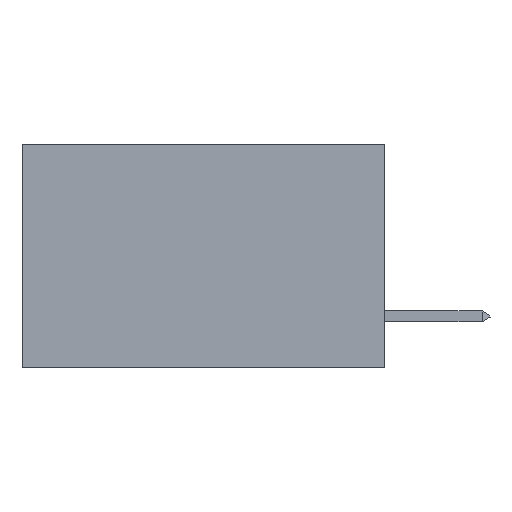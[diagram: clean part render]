
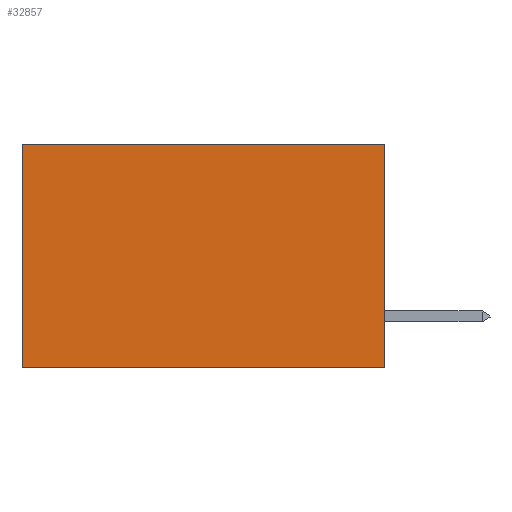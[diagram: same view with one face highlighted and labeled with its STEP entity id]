
A CAD part, left-side view. The second image highlights one B-rep face of the part: STEP entity #32857.
In plain terms, the highlighted planar face has unit normal (-1, 0, 0).
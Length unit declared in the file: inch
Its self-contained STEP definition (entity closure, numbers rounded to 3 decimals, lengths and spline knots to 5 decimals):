
#308 = VECTOR ( 'NONE', #38477, 39.37008 ) ;
#876 = DIRECTION ( 'NONE',  ( 0., 1., 0. ) ) ;
#1437 = VECTOR ( 'NONE', #876, 39.37008 ) ;
#1466 = EDGE_LOOP ( 'NONE', ( #39166, #9387, #15727, #19258 ) ) ;
#1691 = VECTOR ( 'NONE', #33856, 39.37008 ) ;
#2645 = FACE_OUTER_BOUND ( 'NONE', #1466, .T. ) ;
#3293 = DIRECTION ( 'NONE',  ( 1., 0., 0. ) ) ;
#8251 = LINE ( 'NONE', #24584, #25226 ) ;
#9387 = ORIENTED_EDGE ( 'NONE', *, *, #37119, .F. ) ;
#9596 = EDGE_CURVE ( 'NONE', #41830, #18982, #40756, .T. ) ;
#13233 = DIRECTION ( 'NONE',  ( 0., 0., -1. ) ) ;
#13760 = CARTESIAN_POINT ( 'NONE',  ( 0.2875, 0.6, 0. ) ) ;
#15646 = CARTESIAN_POINT ( 'NONE',  ( 0.2875, 0., 0. ) ) ;
#15727 = ORIENTED_EDGE ( 'NONE', *, *, #31345, .F. ) ;
#16260 = PLANE ( 'NONE',  #40070 ) ;
#17340 = VERTEX_POINT ( 'NONE', #19663 ) ;
#18982 = VERTEX_POINT ( 'NONE', #34522 ) ;
#19258 = ORIENTED_EDGE ( 'NONE', *, *, #20784, .T. ) ;
#19530 = CARTESIAN_POINT ( 'NONE',  ( 0.2875, 0., 0. ) ) ;
#19663 = CARTESIAN_POINT ( 'NONE',  ( 0.2875, 0., 0. ) ) ;
#20784 = EDGE_CURVE ( 'NONE', #17340, #41830, #8251, .T. ) ;
#21872 = LINE ( 'NONE', #15646, #308 ) ;
#23462 = CARTESIAN_POINT ( 'NONE',  ( 0.2875, 0., -0.37 ) ) ;
#24584 = CARTESIAN_POINT ( 'NONE',  ( 0.2875, 0., 0. ) ) ;
#25226 = VECTOR ( 'NONE', #27603, 39.37008 ) ;
#25519 = VERTEX_POINT ( 'NONE', #37586 ) ;
#27603 = DIRECTION ( 'NONE',  ( 0., 1., 0. ) ) ;
#31345 = EDGE_CURVE ( 'NONE', #17340, #25519, #21872, .T. ) ;
#32857 = ADVANCED_FACE ( 'NONE', ( #2645 ), #16260, .F. ) ;
#33856 = DIRECTION ( 'NONE',  ( 0., 0., -1. ) ) ;
#33904 = CARTESIAN_POINT ( 'NONE',  ( 0.2875, 0.6, 0. ) ) ;
#34329 = LINE ( 'NONE', #23462, #1437 ) ;
#34522 = CARTESIAN_POINT ( 'NONE',  ( 0.2875, 0.6, -0.37 ) ) ;
#37119 = EDGE_CURVE ( 'NONE', #25519, #18982, #34329, .T. ) ;
#37586 = CARTESIAN_POINT ( 'NONE',  ( 0.2875, 0., -0.37 ) ) ;
#38477 = DIRECTION ( 'NONE',  ( 0., 0., -1. ) ) ;
#39166 = ORIENTED_EDGE ( 'NONE', *, *, #9596, .T. ) ;
#40070 = AXIS2_PLACEMENT_3D ( 'NONE', #19530, #3293, #13233 ) ;
#40756 = LINE ( 'NONE', #13760, #1691 ) ;
#41830 = VERTEX_POINT ( 'NONE', #33904 ) ;
